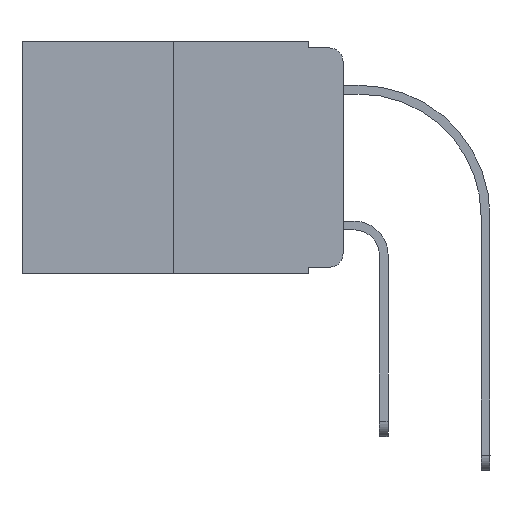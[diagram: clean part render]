
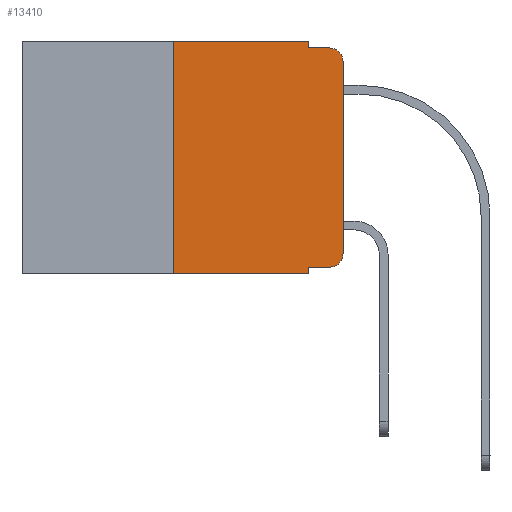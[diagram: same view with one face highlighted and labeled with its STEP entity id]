
A CAD part, left-side view. The second image highlights one B-rep face of the part: STEP entity #13410.
In plain terms, the highlighted planar face has unit normal (-1, 0, 0).
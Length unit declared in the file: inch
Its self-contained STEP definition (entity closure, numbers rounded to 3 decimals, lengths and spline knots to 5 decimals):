
#33 = DIRECTION ( 'NONE',  ( -1., 0., 0. ) ) ;
#122 = EDGE_CURVE ( 'NONE', #9990, #4888, #7505, .T. ) ;
#229 = CARTESIAN_POINT ( 'NONE',  ( 0., 0.051, 0. ) ) ;
#231 = ORIENTED_EDGE ( 'NONE', *, *, #3808, .T. ) ;
#408 = DIRECTION ( 'NONE',  ( 0., -1., 0. ) ) ;
#491 = CARTESIAN_POINT ( 'NONE',  ( 0., 0.051, -0.343 ) ) ;
#536 = VERTEX_POINT ( 'NONE', #12883 ) ;
#568 = CARTESIAN_POINT ( 'NONE',  ( 0., 0.02, -0.01 ) ) ;
#583 = VERTEX_POINT ( 'NONE', #5645 ) ;
#746 = AXIS2_PLACEMENT_3D ( 'NONE', #14576, #33, #2806 ) ;
#809 = VECTOR ( 'NONE', #16534, 39.37008 ) ;
#943 = LINE ( 'NONE', #5076, #9694 ) ;
#1209 = VERTEX_POINT ( 'NONE', #12496 ) ;
#1447 = EDGE_LOOP ( 'NONE', ( #10693, #14349, #4717, #15613, #10592, #14995, #16975, #6260, #231, #15352 ) ) ;
#1700 = CARTESIAN_POINT ( 'NONE',  ( 0., 0.473, -0.343 ) ) ;
#1869 = DIRECTION ( 'NONE',  ( -1., 0., 0. ) ) ;
#2374 = CARTESIAN_POINT ( 'NONE',  ( 0., 0.473, 0. ) ) ;
#2434 = EDGE_CURVE ( 'NONE', #1209, #10281, #15325, .T. ) ;
#2806 = DIRECTION ( 'NONE',  ( 0., 0., -1. ) ) ;
#2834 = CARTESIAN_POINT ( 'NONE',  ( 0., 0., 0. ) ) ;
#2840 = CARTESIAN_POINT ( 'NONE',  ( 0., 0.25, -0.343 ) ) ;
#3039 = DIRECTION ( 'NONE',  ( 0., 0., -1. ) ) ;
#3087 = CARTESIAN_POINT ( 'NONE',  ( 0., 0.051, -0.01 ) ) ;
#3106 = CARTESIAN_POINT ( 'NONE',  ( 0., 0.051, -0.333 ) ) ;
#3808 = EDGE_CURVE ( 'NONE', #14933, #536, #4728, .T. ) ;
#3903 = VECTOR ( 'NONE', #408, 39.37008 ) ;
#4717 = ORIENTED_EDGE ( 'NONE', *, *, #5423, .F. ) ;
#4728 = LINE ( 'NONE', #3106, #9102 ) ;
#4888 = VERTEX_POINT ( 'NONE', #10960 ) ;
#4900 = VECTOR ( 'NONE', #15208, 39.37008 ) ;
#5076 = CARTESIAN_POINT ( 'NONE',  ( 0., 0.25, 0. ) ) ;
#5423 = EDGE_CURVE ( 'NONE', #4888, #10281, #11191, .T. ) ;
#5492 = CARTESIAN_POINT ( 'NONE',  ( 0., 0.02, -0.313 ) ) ;
#5645 = CARTESIAN_POINT ( 'NONE',  ( 0., 0.25, 0. ) ) ;
#5678 = LINE ( 'NONE', #1700, #3903 ) ;
#6021 = CIRCLE ( 'NONE', #12353, 0.02 ) ;
#6220 = DIRECTION ( 'NONE',  ( 0., 0., -1. ) ) ;
#6260 = ORIENTED_EDGE ( 'NONE', *, *, #6394, .F. ) ;
#6394 = EDGE_CURVE ( 'NONE', #14933, #6826, #9756, .T. ) ;
#6826 = VERTEX_POINT ( 'NONE', #491 ) ;
#7167 = EDGE_CURVE ( 'NONE', #583, #9990, #8523, .T. ) ;
#7505 = LINE ( 'NONE', #12746, #8309 ) ;
#7570 = VECTOR ( 'NONE', #9561, 39.37008 ) ;
#8040 = VECTOR ( 'NONE', #11034, 39.37008 ) ;
#8296 = FACE_OUTER_BOUND ( 'NONE', #1447, .T. ) ;
#8309 = VECTOR ( 'NONE', #6220, 39.37008 ) ;
#8431 = CARTESIAN_POINT ( 'NONE',  ( 0., 0., -0.313 ) ) ;
#8509 = DIRECTION ( 'NONE',  ( 0., 0., -1. ) ) ;
#8523 = LINE ( 'NONE', #2374, #8040 ) ;
#8548 = PLANE ( 'NONE',  #15654 ) ;
#9102 = VECTOR ( 'NONE', #9664, 39.37008 ) ;
#9561 = DIRECTION ( 'NONE',  ( 0., 0., 1. ) ) ;
#9602 = CARTESIAN_POINT ( 'NONE',  ( 0., 0.473, 0. ) ) ;
#9664 = DIRECTION ( 'NONE',  ( 0., -1., 0. ) ) ;
#9694 = VECTOR ( 'NONE', #15231, 39.37008 ) ;
#9756 = LINE ( 'NONE', #12323, #809 ) ;
#9990 = VERTEX_POINT ( 'NONE', #229 ) ;
#10034 = EDGE_CURVE ( 'NONE', #15677, #1209, #16173, .T. ) ;
#10269 = CARTESIAN_POINT ( 'NONE',  ( 0., 0.051, -0.333 ) ) ;
#10281 = VERTEX_POINT ( 'NONE', #568 ) ;
#10592 = ORIENTED_EDGE ( 'NONE', *, *, #7167, .F. ) ;
#10693 = ORIENTED_EDGE ( 'NONE', *, *, #10034, .T. ) ;
#10960 = CARTESIAN_POINT ( 'NONE',  ( 0., 0.051, -0.01 ) ) ;
#11034 = DIRECTION ( 'NONE',  ( 0., -1., 0. ) ) ;
#11191 = LINE ( 'NONE', #3087, #4900 ) ;
#12323 = CARTESIAN_POINT ( 'NONE',  ( 0., 0.051, 0. ) ) ;
#12353 = AXIS2_PLACEMENT_3D ( 'NONE', #5492, #1869, #8509 ) ;
#12439 = EDGE_CURVE ( 'NONE', #536, #15677, #6021, .T. ) ;
#12496 = CARTESIAN_POINT ( 'NONE',  ( 0., 0., -0.03 ) ) ;
#12746 = CARTESIAN_POINT ( 'NONE',  ( 0., 0.051, 0. ) ) ;
#12883 = CARTESIAN_POINT ( 'NONE',  ( 0., 0.02, -0.333 ) ) ;
#13410 = ADVANCED_FACE ( 'NONE', ( #8296 ), #8548, .F. ) ;
#14349 = ORIENTED_EDGE ( 'NONE', *, *, #2434, .T. ) ;
#14576 = CARTESIAN_POINT ( 'NONE',  ( 0., 0.02, -0.03 ) ) ;
#14819 = DIRECTION ( 'NONE',  ( 1., 0., 0. ) ) ;
#14933 = VERTEX_POINT ( 'NONE', #10269 ) ;
#14995 = ORIENTED_EDGE ( 'NONE', *, *, #15373, .F. ) ;
#15208 = DIRECTION ( 'NONE',  ( 0., -1., 0. ) ) ;
#15231 = DIRECTION ( 'NONE',  ( 0., 0., 1. ) ) ;
#15325 = CIRCLE ( 'NONE', #746, 0.02 ) ;
#15352 = ORIENTED_EDGE ( 'NONE', *, *, #12439, .T. ) ;
#15373 = EDGE_CURVE ( 'NONE', #15465, #583, #943, .T. ) ;
#15465 = VERTEX_POINT ( 'NONE', #2840 ) ;
#15593 = EDGE_CURVE ( 'NONE', #15465, #6826, #5678, .T. ) ;
#15613 = ORIENTED_EDGE ( 'NONE', *, *, #122, .F. ) ;
#15654 = AXIS2_PLACEMENT_3D ( 'NONE', #9602, #14819, #3039 ) ;
#15677 = VERTEX_POINT ( 'NONE', #8431 ) ;
#16173 = LINE ( 'NONE', #2834, #7570 ) ;
#16534 = DIRECTION ( 'NONE',  ( 0., 0., -1. ) ) ;
#16975 = ORIENTED_EDGE ( 'NONE', *, *, #15593, .T. ) ;
